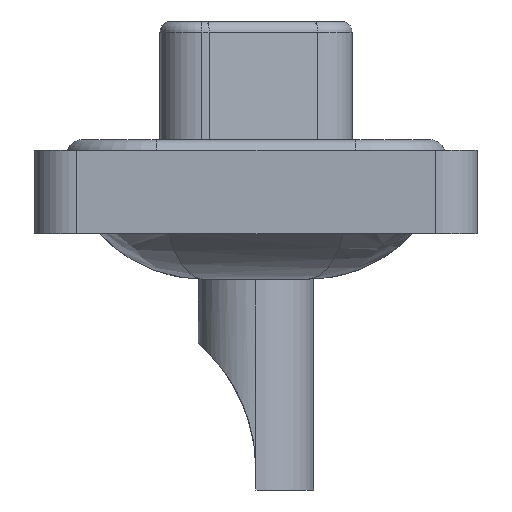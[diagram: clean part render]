
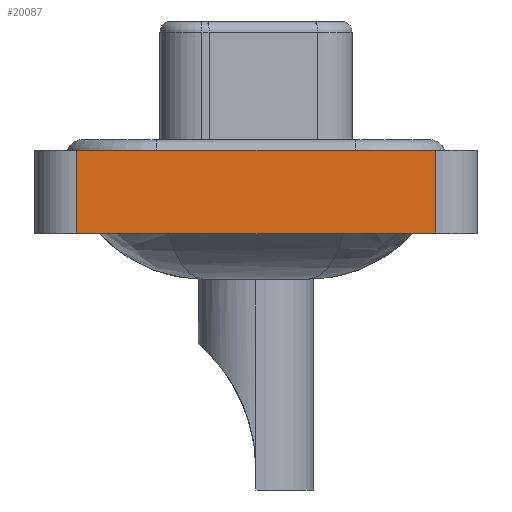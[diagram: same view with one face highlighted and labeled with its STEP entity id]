
A CAD part, left-side view. The second image highlights one B-rep face of the part: STEP entity #20087.
In plain terms, the highlighted planar face has unit normal (-1, 0, 0).
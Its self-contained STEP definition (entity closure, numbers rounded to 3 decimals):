
#1149 = ORIENTED_EDGE ( 'NONE', *, *, #12618, .T. ) ;
#2237 = CARTESIAN_POINT ( 'NONE',  ( -7.35, -8.55, 0.4 ) ) ;
#2512 = LINE ( 'NONE', #3921, #14890 ) ;
#2557 = ORIENTED_EDGE ( 'NONE', *, *, #7170, .T. ) ;
#2649 = LINE ( 'NONE', #4274, #4448 ) ;
#2670 = CARTESIAN_POINT ( 'NONE',  ( -7.35, -8.55, -3.6 ) ) ;
#2822 = VECTOR ( 'NONE', #13770, 1000. ) ;
#3132 = LINE ( 'NONE', #17797, #12541 ) ;
#3695 = EDGE_CURVE ( 'NONE', #15985, #17888, #17236, .T. ) ;
#3921 = CARTESIAN_POINT ( 'NONE',  ( -7.35, -8.55, -3.6 ) ) ;
#4274 = CARTESIAN_POINT ( 'NONE',  ( -7.35, -8.55, 0.4 ) ) ;
#4448 = VECTOR ( 'NONE', #11063, 1000. ) ;
#7170 = EDGE_CURVE ( 'NONE', #18317, #19935, #2512, .T. ) ;
#7714 = DIRECTION ( 'NONE',  ( -1., 0., 0. ) ) ;
#8009 = EDGE_CURVE ( 'NONE', #17888, #19935, #2649, .T. ) ;
#8725 = CARTESIAN_POINT ( 'NONE',  ( -7.35, 8.55, 0.4 ) ) ;
#9449 = PLANE ( 'NONE',  #16831 ) ;
#10975 = FACE_OUTER_BOUND ( 'NONE', #12045, .T. ) ;
#11063 = DIRECTION ( 'NONE',  ( 0., -1., 0. ) ) ;
#11319 = DIRECTION ( 'NONE',  ( 0., -1., 0. ) ) ;
#12045 = EDGE_LOOP ( 'NONE', ( #2557, #17358, #14887, #1149 ) ) ;
#12541 = VECTOR ( 'NONE', #11319, 1000. ) ;
#12618 = EDGE_CURVE ( 'NONE', #15985, #18317, #3132, .T. ) ;
#13770 = DIRECTION ( 'NONE',  ( 0., 0., 1. ) ) ;
#14887 = ORIENTED_EDGE ( 'NONE', *, *, #3695, .F. ) ;
#14890 = VECTOR ( 'NONE', #17304, 1000. ) ;
#15018 = CARTESIAN_POINT ( 'NONE',  ( -7.35, 8.55, -3.6 ) ) ;
#15705 = CARTESIAN_POINT ( 'NONE',  ( -7.35, 8.55, -3.6 ) ) ;
#15985 = VERTEX_POINT ( 'NONE', #15018 ) ;
#16635 = CARTESIAN_POINT ( 'NONE',  ( -7.35, -8.55, -3.6 ) ) ;
#16831 = AXIS2_PLACEMENT_3D ( 'NONE', #2670, #7714, #19271 ) ;
#17236 = LINE ( 'NONE', #15705, #2822 ) ;
#17304 = DIRECTION ( 'NONE',  ( 0., 0., 1. ) ) ;
#17358 = ORIENTED_EDGE ( 'NONE', *, *, #8009, .F. ) ;
#17797 = CARTESIAN_POINT ( 'NONE',  ( -7.35, -8.55, -3.6 ) ) ;
#17888 = VERTEX_POINT ( 'NONE', #8725 ) ;
#18317 = VERTEX_POINT ( 'NONE', #16635 ) ;
#19271 = DIRECTION ( 'NONE',  ( 0., 0., 1. ) ) ;
#19935 = VERTEX_POINT ( 'NONE', #2237 ) ;
#20087 = ADVANCED_FACE ( 'NONE', ( #10975 ), #9449, .T. ) ;
